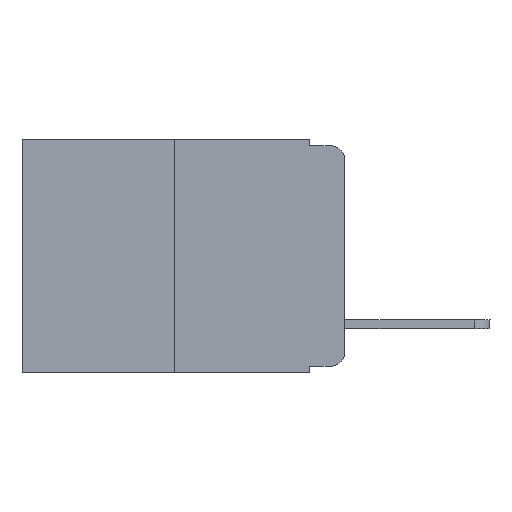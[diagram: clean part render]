
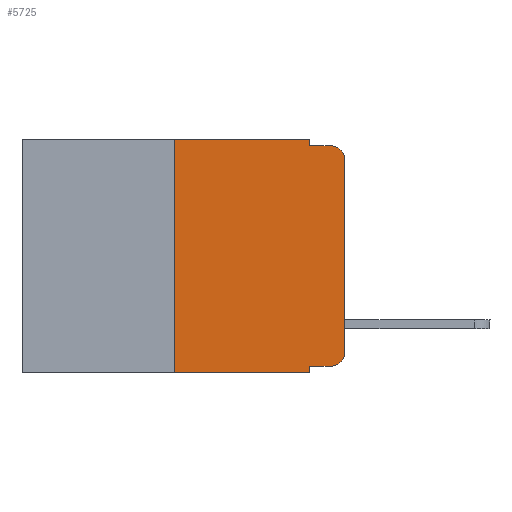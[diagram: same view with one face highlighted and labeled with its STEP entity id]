
A CAD part, left-side view. The second image highlights one B-rep face of the part: STEP entity #5725.
In plain terms, the highlighted planar face has unit normal (-1, 0, 0).
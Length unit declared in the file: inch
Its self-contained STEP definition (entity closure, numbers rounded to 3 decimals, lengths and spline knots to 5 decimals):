
#86 = DIRECTION ( 'NONE',  ( 0., 0., -1. ) ) ;
#233 = DIRECTION ( 'NONE',  ( 0., 0., -1. ) ) ;
#851 = VERTEX_POINT ( 'NONE', #11878 ) ;
#989 = EDGE_CURVE ( 'NONE', #4488, #4564, #6994, .T. ) ;
#1588 = CARTESIAN_POINT ( 'NONE',  ( 0., 0.051, -0.01 ) ) ;
#1628 = DIRECTION ( 'NONE',  ( 0., -1., 0. ) ) ;
#1989 = CARTESIAN_POINT ( 'NONE',  ( 0., 0.473, -0.343 ) ) ;
#2250 = DIRECTION ( 'NONE',  ( -1., 0., 0. ) ) ;
#2278 = ORIENTED_EDGE ( 'NONE', *, *, #22114, .F. ) ;
#2340 = CARTESIAN_POINT ( 'NONE',  ( 0., 0., 0. ) ) ;
#2348 = LINE ( 'NONE', #18503, #2751 ) ;
#2751 = VECTOR ( 'NONE', #18742, 39.37008 ) ;
#3627 = ORIENTED_EDGE ( 'NONE', *, *, #9244, .F. ) ;
#4042 = CARTESIAN_POINT ( 'NONE',  ( 0., 0.02, -0.01 ) ) ;
#4244 = ORIENTED_EDGE ( 'NONE', *, *, #4737, .F. ) ;
#4263 = DIRECTION ( 'NONE',  ( 0., 0., -1. ) ) ;
#4488 = VERTEX_POINT ( 'NONE', #10398 ) ;
#4547 = CARTESIAN_POINT ( 'NONE',  ( 0., 0.051, 0. ) ) ;
#4564 = VERTEX_POINT ( 'NONE', #7065 ) ;
#4658 = CARTESIAN_POINT ( 'NONE',  ( 0., 0.473, 0. ) ) ;
#4737 = EDGE_CURVE ( 'NONE', #4488, #851, #7754, .T. ) ;
#5323 = EDGE_LOOP ( 'NONE', ( #16514, #12584, #16111, #13390, #2278, #3627, #13984, #4244, #14490, #12557 ) ) ;
#5689 = VERTEX_POINT ( 'NONE', #23353 ) ;
#5725 = ADVANCED_FACE ( 'NONE', ( #6950 ), #15883, .F. ) ;
#6404 = EDGE_CURVE ( 'NONE', #20852, #15677, #18271, .T. ) ;
#6582 = CARTESIAN_POINT ( 'NONE',  ( 0., 0.051, 0. ) ) ;
#6604 = EDGE_CURVE ( 'NONE', #7335, #8293, #20503, .T. ) ;
#6716 = CARTESIAN_POINT ( 'NONE',  ( 0., 0.473, 0. ) ) ;
#6833 = DIRECTION ( 'NONE',  ( 1., 0., 0. ) ) ;
#6950 = FACE_OUTER_BOUND ( 'NONE', #5323, .T. ) ;
#6994 = LINE ( 'NONE', #14257, #7684 ) ;
#7065 = CARTESIAN_POINT ( 'NONE',  ( 0., 0.02, -0.333 ) ) ;
#7335 = VERTEX_POINT ( 'NONE', #9773 ) ;
#7582 = CARTESIAN_POINT ( 'NONE',  ( 0., 0.051, 0. ) ) ;
#7684 = VECTOR ( 'NONE', #1628, 39.37008 ) ;
#7717 = CARTESIAN_POINT ( 'NONE',  ( 0., 0.02, -0.313 ) ) ;
#7754 = LINE ( 'NONE', #4547, #22790 ) ;
#8055 = CIRCLE ( 'NONE', #16046, 0.02 ) ;
#8293 = VERTEX_POINT ( 'NONE', #17879 ) ;
#8904 = EDGE_CURVE ( 'NONE', #8293, #22474, #8055, .T. ) ;
#9102 = VECTOR ( 'NONE', #20618, 39.37008 ) ;
#9244 = EDGE_CURVE ( 'NONE', #19190, #5689, #2348, .T. ) ;
#9773 = CARTESIAN_POINT ( 'NONE',  ( 0., 0., -0.313 ) ) ;
#9866 = DIRECTION ( 'NONE',  ( -1., 0., 0. ) ) ;
#9898 = AXIS2_PLACEMENT_3D ( 'NONE', #6716, #6833, #23125 ) ;
#9903 = LINE ( 'NONE', #4658, #19999 ) ;
#10089 = VECTOR ( 'NONE', #15479, 39.37008 ) ;
#10398 = CARTESIAN_POINT ( 'NONE',  ( 0., 0.051, -0.333 ) ) ;
#10504 = VECTOR ( 'NONE', #14270, 39.37008 ) ;
#11160 = LINE ( 'NONE', #1989, #10504 ) ;
#11702 = DIRECTION ( 'NONE',  ( 0., -1., 0. ) ) ;
#11878 = CARTESIAN_POINT ( 'NONE',  ( 0., 0.051, -0.343 ) ) ;
#12557 = ORIENTED_EDGE ( 'NONE', *, *, #18248, .T. ) ;
#12584 = ORIENTED_EDGE ( 'NONE', *, *, #8904, .T. ) ;
#13390 = ORIENTED_EDGE ( 'NONE', *, *, #6404, .F. ) ;
#13464 = DIRECTION ( 'NONE',  ( 0., 0., -1. ) ) ;
#13984 = ORIENTED_EDGE ( 'NONE', *, *, #14808, .T. ) ;
#14257 = CARTESIAN_POINT ( 'NONE',  ( 0., 0.051, -0.333 ) ) ;
#14270 = DIRECTION ( 'NONE',  ( 0., -1., 0. ) ) ;
#14490 = ORIENTED_EDGE ( 'NONE', *, *, #989, .T. ) ;
#14808 = EDGE_CURVE ( 'NONE', #19190, #851, #11160, .T. ) ;
#15366 = CARTESIAN_POINT ( 'NONE',  ( 0., 0.051, -0.01 ) ) ;
#15479 = DIRECTION ( 'NONE',  ( 0., -1., 0. ) ) ;
#15677 = VERTEX_POINT ( 'NONE', #1588 ) ;
#15751 = CIRCLE ( 'NONE', #20279, 0.02 ) ;
#15883 = PLANE ( 'NONE',  #9898 ) ;
#16046 = AXIS2_PLACEMENT_3D ( 'NONE', #18652, #9866, #233 ) ;
#16111 = ORIENTED_EDGE ( 'NONE', *, *, #21057, .F. ) ;
#16466 = CARTESIAN_POINT ( 'NONE',  ( 0., 0.25, -0.343 ) ) ;
#16514 = ORIENTED_EDGE ( 'NONE', *, *, #6604, .T. ) ;
#17879 = CARTESIAN_POINT ( 'NONE',  ( 0., 0., -0.03 ) ) ;
#17892 = VECTOR ( 'NONE', #86, 39.37008 ) ;
#18248 = EDGE_CURVE ( 'NONE', #4564, #7335, #15751, .T. ) ;
#18271 = LINE ( 'NONE', #7582, #17892 ) ;
#18503 = CARTESIAN_POINT ( 'NONE',  ( 0., 0.25, 0. ) ) ;
#18652 = CARTESIAN_POINT ( 'NONE',  ( 0., 0.02, -0.03 ) ) ;
#18742 = DIRECTION ( 'NONE',  ( 0., 0., 1. ) ) ;
#19190 = VERTEX_POINT ( 'NONE', #16466 ) ;
#19999 = VECTOR ( 'NONE', #11702, 39.37008 ) ;
#20279 = AXIS2_PLACEMENT_3D ( 'NONE', #7717, #2250, #4263 ) ;
#20503 = LINE ( 'NONE', #2340, #9102 ) ;
#20618 = DIRECTION ( 'NONE',  ( 0., 0., 1. ) ) ;
#20852 = VERTEX_POINT ( 'NONE', #6582 ) ;
#21057 = EDGE_CURVE ( 'NONE', #15677, #22474, #22613, .T. ) ;
#22114 = EDGE_CURVE ( 'NONE', #5689, #20852, #9903, .T. ) ;
#22474 = VERTEX_POINT ( 'NONE', #4042 ) ;
#22613 = LINE ( 'NONE', #15366, #10089 ) ;
#22790 = VECTOR ( 'NONE', #13464, 39.37008 ) ;
#23125 = DIRECTION ( 'NONE',  ( 0., 0., -1. ) ) ;
#23353 = CARTESIAN_POINT ( 'NONE',  ( 0., 0.25, 0. ) ) ;
